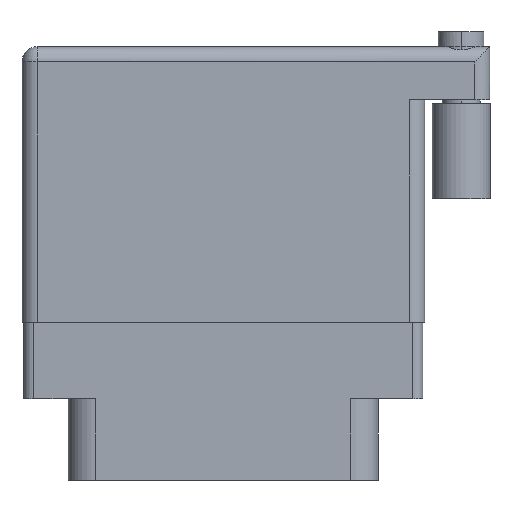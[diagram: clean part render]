
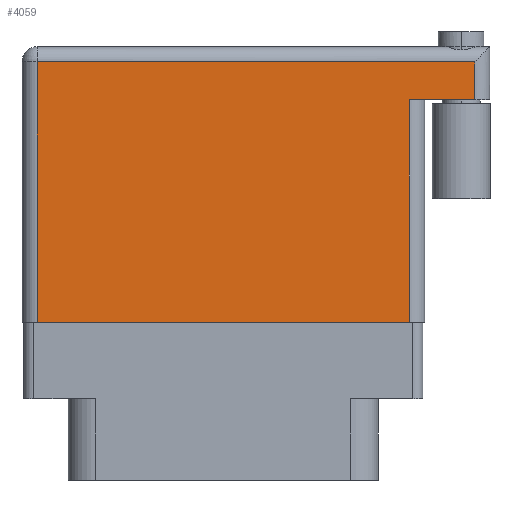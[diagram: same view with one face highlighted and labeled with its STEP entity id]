
A CAD part, front view. The second image highlights one B-rep face of the part: STEP entity #4059.
In plain terms, the highlighted face is planar.
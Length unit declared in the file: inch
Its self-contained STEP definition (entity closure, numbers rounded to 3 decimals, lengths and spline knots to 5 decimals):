
#1247 = EDGE_LOOP ( 'NONE', ( #11924, #17243, #5628, #21491, #20886, #12632 ) ) ;
#1558 = EDGE_CURVE ( 'NONE', #20525, #3770, #21190, .T. ) ;
#1634 = DIRECTION ( 'NONE',  ( 0., 1., 0. ) ) ;
#1643 = LINE ( 'NONE', #20314, #11331 ) ;
#1706 = EDGE_CURVE ( 'NONE', #20525, #7867, #3310, .T. ) ;
#3266 = CARTESIAN_POINT ( 'NONE',  ( 0.05, 0., 0. ) ) ;
#3305 = EDGE_CURVE ( 'NONE', #9648, #3770, #13304, .T. ) ;
#3310 = LINE ( 'NONE', #14988, #7654 ) ;
#3770 = VERTEX_POINT ( 'NONE', #8798 ) ;
#4059 = ADVANCED_FACE ( 'NONE', ( #17068 ), #20392, .F. ) ;
#4729 = EDGE_CURVE ( 'NONE', #7867, #15991, #1643, .T. ) ;
#5628 = ORIENTED_EDGE ( 'NONE', *, *, #1558, .F. ) ;
#6243 = CARTESIAN_POINT ( 'NONE',  ( 0.05, 0.856, 0. ) ) ;
#7121 = VECTOR ( 'NONE', #18286, 39.37008 ) ;
#7654 = VECTOR ( 'NONE', #1634, 39.37008 ) ;
#7867 = VERTEX_POINT ( 'NONE', #19079 ) ;
#8798 = CARTESIAN_POINT ( 'NONE',  ( 1.275, 0.731, 0. ) ) ;
#8942 = DIRECTION ( 'NONE',  ( 0., 0., -1. ) ) ;
#9470 = LINE ( 'NONE', #9584, #17589 ) ;
#9584 = CARTESIAN_POINT ( 'NONE',  ( 0., 0., 0. ) ) ;
#9648 = VERTEX_POINT ( 'NONE', #17938 ) ;
#11154 = EDGE_CURVE ( 'NONE', #19937, #9648, #9470, .T. ) ;
#11331 = VECTOR ( 'NONE', #15218, 39.37008 ) ;
#11527 = CARTESIAN_POINT ( 'NONE',  ( 1.275, 0.731, 0. ) ) ;
#11612 = DIRECTION ( 'NONE',  ( 0., -1., 0. ) ) ;
#11924 = ORIENTED_EDGE ( 'NONE', *, *, #11154, .T. ) ;
#12589 = DIRECTION ( 'NONE',  ( 1., 0., 0. ) ) ;
#12632 = ORIENTED_EDGE ( 'NONE', *, *, #12905, .T. ) ;
#12905 = EDGE_CURVE ( 'NONE', #15991, #19937, #18489, .T. ) ;
#13304 = LINE ( 'NONE', #11527, #7121 ) ;
#14988 = CARTESIAN_POINT ( 'NONE',  ( 1.489, 0.906, 0. ) ) ;
#15038 = CARTESIAN_POINT ( 'NONE',  ( 0.05, 0., 0. ) ) ;
#15218 = DIRECTION ( 'NONE',  ( -1., 0., 0. ) ) ;
#15351 = VECTOR ( 'NONE', #11612, 39.37008 ) ;
#15991 = VERTEX_POINT ( 'NONE', #6243 ) ;
#17068 = FACE_OUTER_BOUND ( 'NONE', #1247, .T. ) ;
#17171 = CARTESIAN_POINT ( 'NONE',  ( 0., 0.906, 0. ) ) ;
#17243 = ORIENTED_EDGE ( 'NONE', *, *, #3305, .T. ) ;
#17589 = VECTOR ( 'NONE', #12589, 39.37008 ) ;
#17938 = CARTESIAN_POINT ( 'NONE',  ( 1.275, 0., 0. ) ) ;
#17967 = DIRECTION ( 'NONE',  ( -1., 0., 0. ) ) ;
#18286 = DIRECTION ( 'NONE',  ( 0., 1., 0. ) ) ;
#18489 = LINE ( 'NONE', #3266, #15351 ) ;
#18944 = DIRECTION ( 'NONE',  ( -1., 0., 0. ) ) ;
#19051 = CARTESIAN_POINT ( 'NONE',  ( 1.489, 0.731, 0. ) ) ;
#19079 = CARTESIAN_POINT ( 'NONE',  ( 1.489, 0.856, 0. ) ) ;
#19278 = AXIS2_PLACEMENT_3D ( 'NONE', #17171, #8942, #18944 ) ;
#19937 = VERTEX_POINT ( 'NONE', #15038 ) ;
#20314 = CARTESIAN_POINT ( 'NONE',  ( 0., 0.856, 0. ) ) ;
#20392 = PLANE ( 'NONE',  #19278 ) ;
#20525 = VERTEX_POINT ( 'NONE', #19051 ) ;
#20886 = ORIENTED_EDGE ( 'NONE', *, *, #4729, .T. ) ;
#21190 = LINE ( 'NONE', #21419, #21488 ) ;
#21419 = CARTESIAN_POINT ( 'NONE',  ( 1.539, 0.731, 0. ) ) ;
#21488 = VECTOR ( 'NONE', #17967, 39.37008 ) ;
#21491 = ORIENTED_EDGE ( 'NONE', *, *, #1706, .T. ) ;
